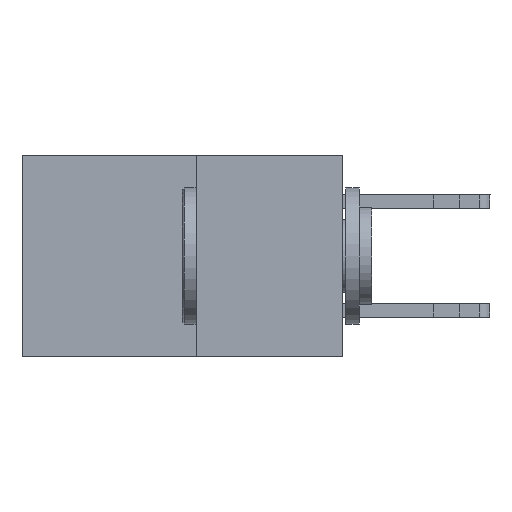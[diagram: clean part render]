
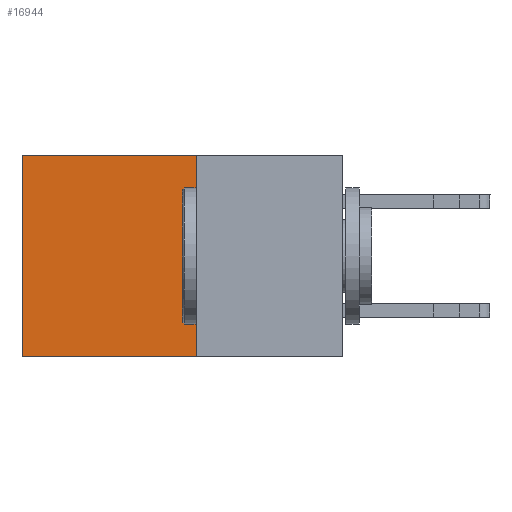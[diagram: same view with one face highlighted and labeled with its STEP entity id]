
A CAD part, left-side view. The second image highlights one B-rep face of the part: STEP entity #16944.
In plain terms, the highlighted planar face has unit normal (-1, 0, 0).
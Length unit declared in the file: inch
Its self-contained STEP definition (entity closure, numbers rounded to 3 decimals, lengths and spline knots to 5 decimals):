
#445 = VECTOR ( 'NONE', #22198, 39.37008 ) ;
#4735 = CARTESIAN_POINT ( 'NONE',  ( 0.277, 0.27, -0.37 ) ) ;
#5581 = EDGE_CURVE ( 'NONE', #17298, #14631, #11798, .T. ) ;
#5894 = DIRECTION ( 'NONE',  ( 1., 0., 0. ) ) ;
#7649 = DIRECTION ( 'NONE',  ( 0., 0., -1. ) ) ;
#7773 = PLANE ( 'NONE',  #25913 ) ;
#8443 = VECTOR ( 'NONE', #18671, 39.37008 ) ;
#8760 = CARTESIAN_POINT ( 'NONE',  ( 0.277, 0.59, -0.37 ) ) ;
#9444 = ORIENTED_EDGE ( 'NONE', *, *, #5581, .T. ) ;
#9711 = CARTESIAN_POINT ( 'NONE',  ( 0.277, 0.59, 0. ) ) ;
#11356 = ORIENTED_EDGE ( 'NONE', *, *, #26448, .T. ) ;
#11526 = FACE_OUTER_BOUND ( 'NONE', #12535, .T. ) ;
#11798 = LINE ( 'NONE', #24302, #15301 ) ;
#12535 = EDGE_LOOP ( 'NONE', ( #9444, #14332, #13543, #11356 ) ) ;
#13543 = ORIENTED_EDGE ( 'NONE', *, *, #23537, .F. ) ;
#14332 = ORIENTED_EDGE ( 'NONE', *, *, #19757, .F. ) ;
#14631 = VERTEX_POINT ( 'NONE', #8760 ) ;
#15301 = VECTOR ( 'NONE', #19744, 39.37008 ) ;
#16039 = CARTESIAN_POINT ( 'NONE',  ( 0.277, 0.27, 0. ) ) ;
#16944 = ADVANCED_FACE ( 'NONE', ( #11526 ), #7773, .F. ) ;
#17298 = VERTEX_POINT ( 'NONE', #9711 ) ;
#17851 = VERTEX_POINT ( 'NONE', #24320 ) ;
#18651 = LINE ( 'NONE', #24850, #23375 ) ;
#18671 = DIRECTION ( 'NONE',  ( 0., 1., 0. ) ) ;
#19744 = DIRECTION ( 'NONE',  ( 0., 0., -1. ) ) ;
#19757 = EDGE_CURVE ( 'NONE', #17851, #14631, #20836, .T. ) ;
#20836 = LINE ( 'NONE', #4735, #8443 ) ;
#21804 = CARTESIAN_POINT ( 'NONE',  ( 0.277, 0.27, -0.37 ) ) ;
#22198 = DIRECTION ( 'NONE',  ( 0., 0., -1. ) ) ;
#22255 = VERTEX_POINT ( 'NONE', #16039 ) ;
#23375 = VECTOR ( 'NONE', #24967, 39.37008 ) ;
#23537 = EDGE_CURVE ( 'NONE', #22255, #17851, #24343, .T. ) ;
#24282 = CARTESIAN_POINT ( 'NONE',  ( 0.277, 0.27, -0.37 ) ) ;
#24302 = CARTESIAN_POINT ( 'NONE',  ( 0.277, 0.59, -0.37 ) ) ;
#24320 = CARTESIAN_POINT ( 'NONE',  ( 0.277, 0.27, -0.37 ) ) ;
#24343 = LINE ( 'NONE', #21804, #445 ) ;
#24850 = CARTESIAN_POINT ( 'NONE',  ( 0.277, 0.27, 0. ) ) ;
#24967 = DIRECTION ( 'NONE',  ( 0., 1., 0. ) ) ;
#25913 = AXIS2_PLACEMENT_3D ( 'NONE', #24282, #5894, #7649 ) ;
#26448 = EDGE_CURVE ( 'NONE', #22255, #17298, #18651, .T. ) ;
